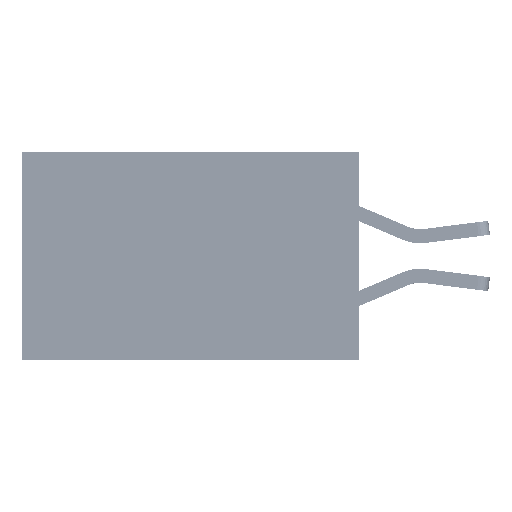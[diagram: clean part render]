
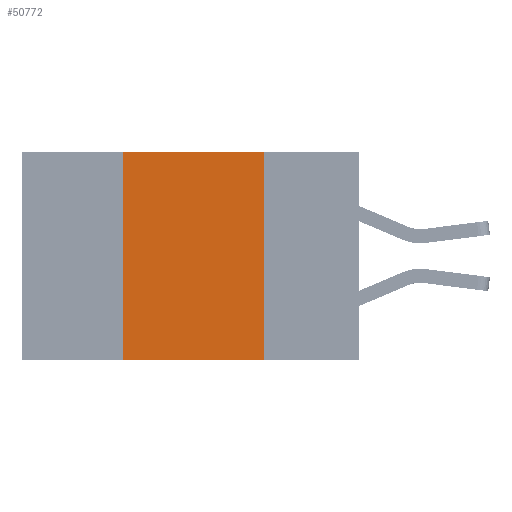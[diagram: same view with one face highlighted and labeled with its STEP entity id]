
A CAD part, left-side view. The second image highlights one B-rep face of the part: STEP entity #50772.
In plain terms, the highlighted planar face has unit normal (-1, 0, 0).
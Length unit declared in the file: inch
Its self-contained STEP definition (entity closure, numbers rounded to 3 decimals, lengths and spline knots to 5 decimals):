
#124 = CARTESIAN_POINT ( 'NONE',  ( 0., 0.6, -0.37 ) ) ;
#2540 = EDGE_CURVE ( 'NONE', #25859, #3586, #36027, .T. ) ;
#3586 = VERTEX_POINT ( 'NONE', #29273 ) ;
#6103 = ORIENTED_EDGE ( 'NONE', *, *, #50313, .F. ) ;
#7661 = EDGE_LOOP ( 'NONE', ( #48611, #6103, #49290, #38177 ) ) ;
#7800 = VECTOR ( 'NONE', #48454, 39.37008 ) ;
#11506 = VECTOR ( 'NONE', #36239, 39.37008 ) ;
#16596 = PLANE ( 'NONE',  #39057 ) ;
#18101 = CARTESIAN_POINT ( 'NONE',  ( 0., 0.6, 0. ) ) ;
#18113 = CARTESIAN_POINT ( 'NONE',  ( 0., 0.17, 0. ) ) ;
#18552 = LINE ( 'NONE', #32152, #11506 ) ;
#22366 = VERTEX_POINT ( 'NONE', #18113 ) ;
#22470 = LINE ( 'NONE', #18101, #30163 ) ;
#25859 = VERTEX_POINT ( 'NONE', #44556 ) ;
#25866 = VECTOR ( 'NONE', #31153, 39.37008 ) ;
#29273 = CARTESIAN_POINT ( 'NONE',  ( 0., 0.42, 0. ) ) ;
#29546 = EDGE_CURVE ( 'NONE', #22366, #51042, #18552, .T. ) ;
#30163 = VECTOR ( 'NONE', #46626, 39.37008 ) ;
#31153 = DIRECTION ( 'NONE',  ( 0., 0., 1. ) ) ;
#32152 = CARTESIAN_POINT ( 'NONE',  ( 0., 0.17, 0. ) ) ;
#33922 = DIRECTION ( 'NONE',  ( 1., 0., 0. ) ) ;
#34275 = CARTESIAN_POINT ( 'NONE',  ( 0., 0.6, 0. ) ) ;
#35263 = CARTESIAN_POINT ( 'NONE',  ( 0., 0.42, 0. ) ) ;
#36027 = LINE ( 'NONE', #35263, #25866 ) ;
#36239 = DIRECTION ( 'NONE',  ( 0., 0., -1. ) ) ;
#37093 = FACE_OUTER_BOUND ( 'NONE', #7661, .T. ) ;
#38177 = ORIENTED_EDGE ( 'NONE', *, *, #41079, .T. ) ;
#39057 = AXIS2_PLACEMENT_3D ( 'NONE', #34275, #33922, #50107 ) ;
#41079 = EDGE_CURVE ( 'NONE', #25859, #51042, #51225, .T. ) ;
#44556 = CARTESIAN_POINT ( 'NONE',  ( 0., 0.42, -0.37 ) ) ;
#46626 = DIRECTION ( 'NONE',  ( 0., -1., 0. ) ) ;
#47934 = CARTESIAN_POINT ( 'NONE',  ( 0., 0.17, -0.37 ) ) ;
#48454 = DIRECTION ( 'NONE',  ( 0., -1., 0. ) ) ;
#48611 = ORIENTED_EDGE ( 'NONE', *, *, #29546, .F. ) ;
#49290 = ORIENTED_EDGE ( 'NONE', *, *, #2540, .F. ) ;
#50107 = DIRECTION ( 'NONE',  ( 0., 0., -1. ) ) ;
#50313 = EDGE_CURVE ( 'NONE', #3586, #22366, #22470, .T. ) ;
#50772 = ADVANCED_FACE ( 'NONE', ( #37093 ), #16596, .F. ) ;
#51042 = VERTEX_POINT ( 'NONE', #47934 ) ;
#51225 = LINE ( 'NONE', #124, #7800 ) ;
